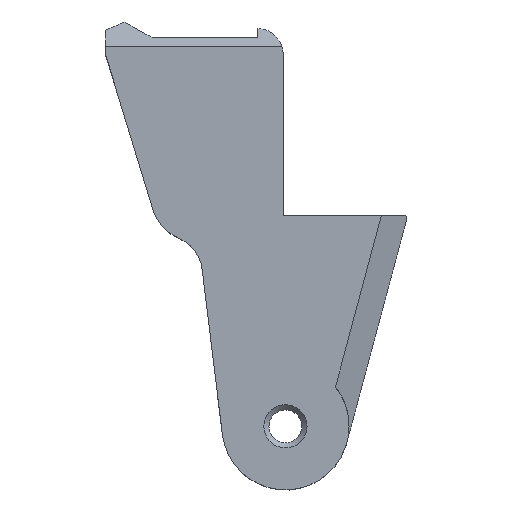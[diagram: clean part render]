
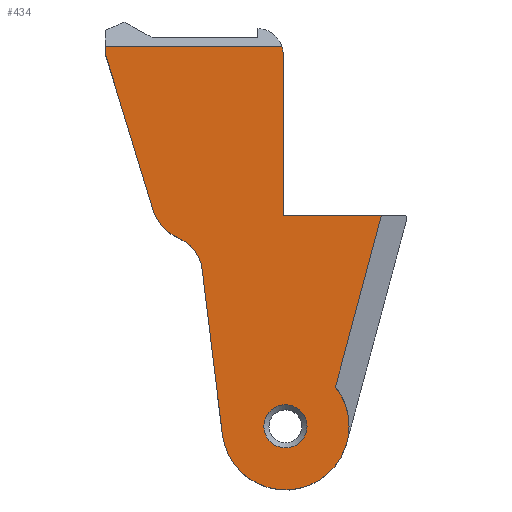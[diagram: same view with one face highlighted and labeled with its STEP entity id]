
A CAD part, top view. The second image highlights one B-rep face of the part: STEP entity #434.
In plain terms, the highlighted planar face has unit normal (0, 0, 1).
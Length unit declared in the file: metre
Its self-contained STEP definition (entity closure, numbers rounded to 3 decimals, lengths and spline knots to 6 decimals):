
#34=CIRCLE('',#476,0.00635);
#35=CIRCLE('',#480,0.00254);
#38=CIRCLE('',#487,0.002159);
#39=CIRCLE('',#488,0.004775);
#40=CIRCLE('',#489,0.00381);
#113=ORIENTED_EDGE('',*,*,#215,.T.);
#114=ORIENTED_EDGE('',*,*,#165,.T.);
#115=ORIENTED_EDGE('',*,*,#216,.T.);
#116=ORIENTED_EDGE('',*,*,#217,.F.);
#117=ORIENTED_EDGE('',*,*,#218,.F.);
#118=ORIENTED_EDGE('',*,*,#199,.F.);
#119=ORIENTED_EDGE('',*,*,#219,.T.);
#120=ORIENTED_EDGE('',*,*,#212,.F.);
#121=ORIENTED_EDGE('',*,*,#207,.T.);
#122=ORIENTED_EDGE('',*,*,#205,.F.);
#123=ORIENTED_EDGE('',*,*,#189,.T.);
#124=ORIENTED_EDGE('',*,*,#202,.T.);
#165=EDGE_CURVE('',#227,#226,#268,.T.);
#189=EDGE_CURVE('',#247,#246,#284,.T.);
#199=EDGE_CURVE('',#254,#255,#34,.T.);
#202=EDGE_CURVE('',#246,#227,#293,.T.);
#205=EDGE_CURVE('',#247,#256,#35,.T.);
#207=EDGE_CURVE('',#257,#256,#297,.T.);
#212=EDGE_CURVE('',#257,#258,#302,.T.);
#215=EDGE_CURVE('',#263,#263,#38,.T.);
#216=EDGE_CURVE('',#226,#264,#39,.F.);
#217=EDGE_CURVE('',#265,#264,#40,.T.);
#218=EDGE_CURVE('',#255,#265,#303,.T.);
#219=EDGE_CURVE('',#254,#258,#304,.T.);
#226=VERTEX_POINT('',#639);
#227=VERTEX_POINT('',#641);
#246=VERTEX_POINT('',#687);
#247=VERTEX_POINT('',#689);
#254=VERTEX_POINT('',#707);
#255=VERTEX_POINT('',#709);
#256=VERTEX_POINT('',#719);
#257=VERTEX_POINT('',#723);
#258=VERTEX_POINT('',#727);
#263=VERTEX_POINT('',#740);
#264=VERTEX_POINT('',#742);
#265=VERTEX_POINT('',#744);
#268=LINE('',#640,#309);
#284=LINE('',#688,#325);
#293=LINE('',#713,#334);
#297=LINE('',#722,#338);
#302=LINE('',#732,#343);
#303=LINE('',#745,#344);
#304=LINE('',#746,#345);
#309=VECTOR('',#508,1.);
#325=VECTOR('',#548,1.);
#334=VECTOR('',#571,1.);
#338=VECTOR('',#583,1.);
#343=VECTOR('',#590,1.);
#344=VECTOR('',#605,1.);
#345=VECTOR('',#606,1.);
#363=EDGE_LOOP('',(#113));
#364=EDGE_LOOP('',(#114,#115,#116,#117,#118,#119,#120,#121,#122,#123,#124));
#392=FACE_BOUND('',#363,.T.);
#393=FACE_BOUND('',#364,.T.);
#416=PLANE('',#486);
#434=ADVANCED_FACE('',(#392,#393),#416,.F.);
#476=AXIS2_PLACEMENT_3D('',#708,#565,#566);
#480=AXIS2_PLACEMENT_3D('',#718,#578,#579);
#486=AXIS2_PLACEMENT_3D('',#738,#597,#598);
#487=AXIS2_PLACEMENT_3D('',#739,#599,#600);
#488=AXIS2_PLACEMENT_3D('',#741,#601,#602);
#489=AXIS2_PLACEMENT_3D('',#743,#603,#604);
#508=DIRECTION('',(0.292,-0.957,0.));
#548=DIRECTION('',(-1.,0.,0.));
#565=DIRECTION('',(0.,0.,-1.));
#566=DIRECTION('',(-1.,0.,0.));
#571=DIRECTION('',(0.,-1.,0.));
#578=DIRECTION('',(0.,0.,-1.));
#579=DIRECTION('',(-1.,0.,0.));
#583=DIRECTION('',(0.,1.,0.));
#590=DIRECTION('',(1.,0.,0.));
#597=DIRECTION('',(0.,0.,-1.));
#598=DIRECTION('',(1.,0.,0.));
#599=DIRECTION('',(0.,0.,-1.));
#600=DIRECTION('',(-1.,0.,0.));
#601=DIRECTION('',(0.,0.,-1.));
#602=DIRECTION('',(-1.,0.,0.));
#603=DIRECTION('',(0.,0.,1.));
#604=DIRECTION('',(1.,0.,0.));
#605=DIRECTION('',(-0.121,0.993,0.));
#606=DIRECTION('',(0.259,0.966,0.));
#639=CARTESIAN_POINT('',(-0.011678,0.018053,0.));
#640=CARTESIAN_POINT('',(-0.010454,0.01404,0.));
#641=CARTESIAN_POINT('',(-0.016421,0.033611,0.));
#687=CARTESIAN_POINT('',(-0.016421,0.034246,0.));
#688=CARTESIAN_POINT('',(-0.007704,0.034246,0.));
#689=CARTESIAN_POINT('',(0.001242,0.034246,0.));
#707=CARTESIAN_POINT('',(0.006583,0.000243,0.));
#708=CARTESIAN_POINT('',(0.001588,-0.003678,0.));
#709=CARTESIAN_POINT('',(-0.004715,-0.004447,0.));
#713=CARTESIAN_POINT('',(-0.016421,0.035198,0.));
#718=CARTESIAN_POINT('',(-0.001181,0.033484,0.));
#719=CARTESIAN_POINT('',(0.001359,0.033484,0.));
#722=CARTESIAN_POINT('',(0.001359,0.042022,0.));
#723=CARTESIAN_POINT('',(0.001359,0.017365,0.));
#727=CARTESIAN_POINT('',(0.011171,0.017365,0.));
#732=CARTESIAN_POINT('',(0.01715,0.017365,0.));
#738=CARTESIAN_POINT('',(-0.007704,0.001813,0.));
#739=CARTESIAN_POINT('',(0.001588,-0.003678,0.));
#740=CARTESIAN_POINT('',(-0.000571,-0.003678,0.));
#741=CARTESIAN_POINT('',(-0.00711,0.019446,0.));
#742=CARTESIAN_POINT('',(-0.009,0.015061,0.));
#743=CARTESIAN_POINT('',(-0.010507,0.011562,0.));
#744=CARTESIAN_POINT('',(-0.006726,0.012023,0.));
#745=CARTESIAN_POINT('',(-0.00572,0.003788,0.));
#746=CARTESIAN_POINT('',(0.011347,0.018023,0.));
